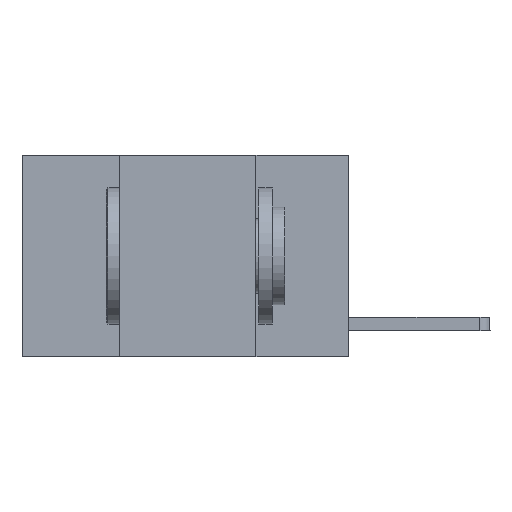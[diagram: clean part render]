
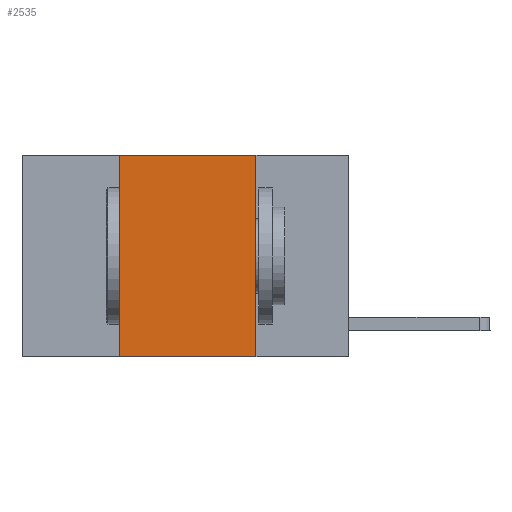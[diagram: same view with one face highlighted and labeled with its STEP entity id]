
A CAD part, left-side view. The second image highlights one B-rep face of the part: STEP entity #2535.
In plain terms, the highlighted planar face has unit normal (-1, 0, 0).
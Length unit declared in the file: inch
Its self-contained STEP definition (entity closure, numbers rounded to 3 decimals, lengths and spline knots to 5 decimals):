
#156 = AXIS2_PLACEMENT_3D ( 'NONE', #4172, #5654, #7210 ) ;
#489 = DIRECTION ( 'NONE',  ( 0., -1., 0. ) ) ;
#602 = VECTOR ( 'NONE', #8776, 39.37008 ) ;
#644 = CARTESIAN_POINT ( 'NONE',  ( 0., 0.17, 0. ) ) ;
#745 = CARTESIAN_POINT ( 'NONE',  ( 0., 0.17, -0.37 ) ) ;
#1288 = DIRECTION ( 'NONE',  ( 0., 0., 1. ) ) ;
#1323 = EDGE_CURVE ( 'NONE', #8337, #1439, #6953, .T. ) ;
#1439 = VERTEX_POINT ( 'NONE', #745 ) ;
#2082 = LINE ( 'NONE', #8731, #3738 ) ;
#2239 = DIRECTION ( 'NONE',  ( 0., 0., -1. ) ) ;
#2535 = ADVANCED_FACE ( 'NONE', ( #3406 ), #5746, .F. ) ;
#2834 = CARTESIAN_POINT ( 'NONE',  ( 0., 0.17, 0. ) ) ;
#2983 = EDGE_CURVE ( 'NONE', #6572, #8337, #2082, .T. ) ;
#3406 = FACE_OUTER_BOUND ( 'NONE', #9224, .T. ) ;
#3543 = ORIENTED_EDGE ( 'NONE', *, *, #2983, .F. ) ;
#3738 = VECTOR ( 'NONE', #489, 39.37008 ) ;
#4165 = VECTOR ( 'NONE', #1288, 39.37008 ) ;
#4172 = CARTESIAN_POINT ( 'NONE',  ( 0., 0.6, 0. ) ) ;
#5654 = DIRECTION ( 'NONE',  ( 1., 0., 0. ) ) ;
#5746 = PLANE ( 'NONE',  #156 ) ;
#5999 = VECTOR ( 'NONE', #2239, 39.37008 ) ;
#6028 = VERTEX_POINT ( 'NONE', #6996 ) ;
#6065 = ORIENTED_EDGE ( 'NONE', *, *, #6137, .F. ) ;
#6137 = EDGE_CURVE ( 'NONE', #6028, #6572, #7985, .T. ) ;
#6572 = VERTEX_POINT ( 'NONE', #8275 ) ;
#6953 = LINE ( 'NONE', #644, #5999 ) ;
#6996 = CARTESIAN_POINT ( 'NONE',  ( 0., 0.42, -0.37 ) ) ;
#7083 = CARTESIAN_POINT ( 'NONE',  ( 0., 0.6, -0.37 ) ) ;
#7084 = ORIENTED_EDGE ( 'NONE', *, *, #8741, .T. ) ;
#7210 = DIRECTION ( 'NONE',  ( 0., 0., -1. ) ) ;
#7248 = CARTESIAN_POINT ( 'NONE',  ( 0., 0.42, 0. ) ) ;
#7985 = LINE ( 'NONE', #7248, #4165 ) ;
#8275 = CARTESIAN_POINT ( 'NONE',  ( 0., 0.42, 0. ) ) ;
#8337 = VERTEX_POINT ( 'NONE', #2834 ) ;
#8731 = CARTESIAN_POINT ( 'NONE',  ( 0., 0.6, 0. ) ) ;
#8741 = EDGE_CURVE ( 'NONE', #6028, #1439, #9311, .T. ) ;
#8776 = DIRECTION ( 'NONE',  ( 0., -1., 0. ) ) ;
#9224 = EDGE_LOOP ( 'NONE', ( #9619, #3543, #6065, #7084 ) ) ;
#9311 = LINE ( 'NONE', #7083, #602 ) ;
#9619 = ORIENTED_EDGE ( 'NONE', *, *, #1323, .F. ) ;
